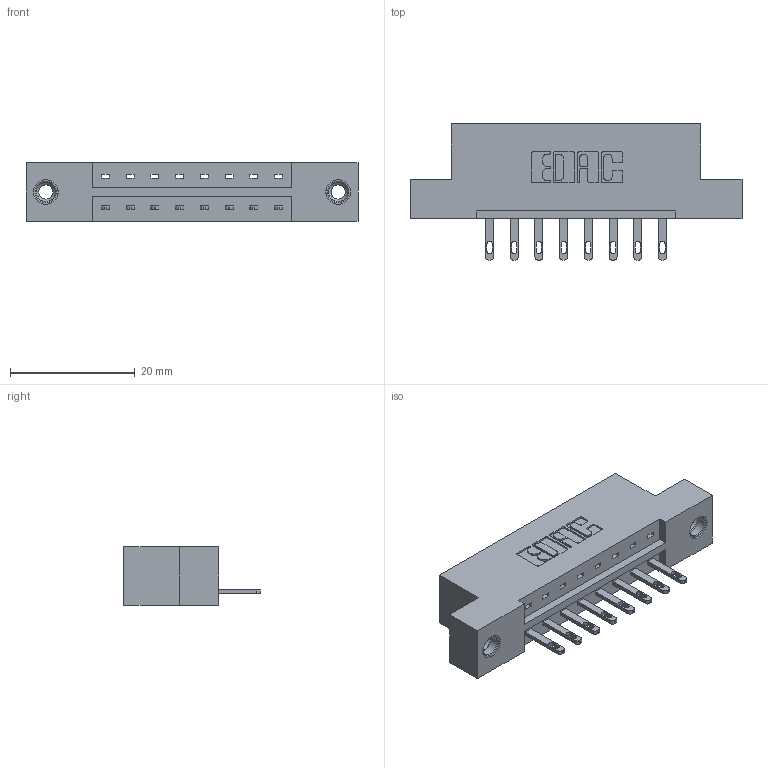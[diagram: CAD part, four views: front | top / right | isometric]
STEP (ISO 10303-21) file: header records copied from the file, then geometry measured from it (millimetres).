
FILE_DESCRIPTION (( 'STEP AP203' ), '1' );
FILE_NAME ('833-008-500-108.STEP', '2020-05-30T15:35:18', ( '' ), ( '' ), 'SwSTEP 2.0', 'SolidWorks 2020', '' );
FILE_SCHEMA (( 'CONFIG_CONTROL_DESIGN' ));
Length unit declared in the file: inch
Products named in the file (4): 345-250-001_345-250-003-102; 833-008-500-108; 833 Part_Flush - .156 Dia - TI; 345-292-001_345-293-100
Assembly tree (11 placements, depth 2):
  833-008-500-108
    833 Part_Flush - .156 Dia - TI
    345-292-001_345-293-100  x8
    345-250-001_345-250-003-102  x2
Bounding box: 53.24 x 21.85 x 9.4 mm (x, y, z)
Volume: 5063.3 mm3; surface area: 5301.1 mm2
Topology: 11 solids, 11 shells, 606 faces, 1791 edges, 1186 vertices
Faces by surface type: plane 390, cylinder 200, cone 12, torus 4
Entity records: 10404 total; most frequent: CARTESIAN_POINT 1781, ORIENTED_EDGE 1718, DIRECTION 1605, EDGE_CURVE 859, VECTOR 707, LINE 707, VERTEX_POINT 568, AXIS2_PLACEMENT_3D 449
